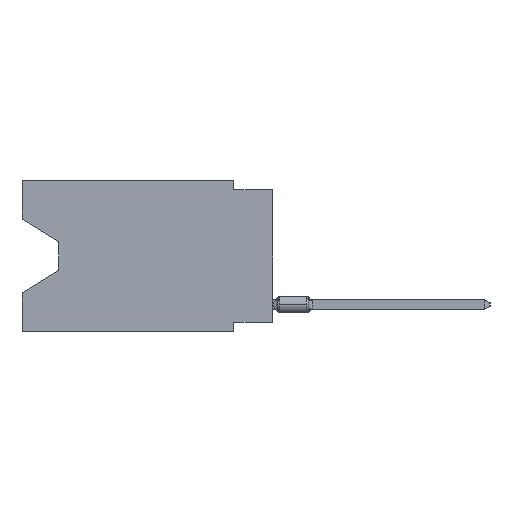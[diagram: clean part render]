
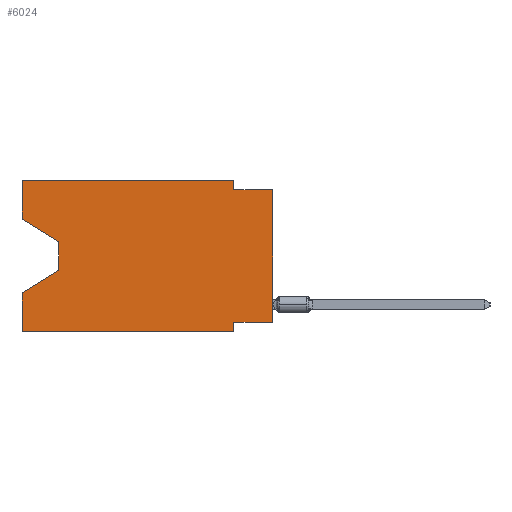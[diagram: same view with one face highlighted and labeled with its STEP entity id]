
A CAD part, left-side view. The second image highlights one B-rep face of the part: STEP entity #6024.
In plain terms, the highlighted planar face has unit normal (-1, 0, 0).
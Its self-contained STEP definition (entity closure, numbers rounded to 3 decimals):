
#334 = ORIENTED_EDGE ( 'NONE', *, *, #66144, .F. ) ;
#1323 = CARTESIAN_POINT ( 'NONE',  ( 0., 16.383, 0. ) ) ;
#2245 = VECTOR ( 'NONE', #31888, 1000. ) ;
#2262 = CARTESIAN_POINT ( 'NONE',  ( 0., 0., -9.271 ) ) ;
#2269 = CARTESIAN_POINT ( 'NONE',  ( 0., 0., -9.271 ) ) ;
#2447 = DIRECTION ( 'NONE',  ( 0., -1., 0. ) ) ;
#5478 = VECTOR ( 'NONE', #59322, 1000. ) ;
#5703 = DIRECTION ( 'NONE',  ( 0., 0.855, -0.519 ) ) ;
#5725 = EDGE_CURVE ( 'NONE', #48758, #46616, #27252, .T. ) ;
#6010 = CARTESIAN_POINT ( 'NONE',  ( 0., 2.54, 0. ) ) ;
#6024 = ADVANCED_FACE ( 'NONE', ( #52932 ), #61983, .F. ) ;
#7100 = CARTESIAN_POINT ( 'NONE',  ( 0., 16.383, -2.546 ) ) ;
#7611 = VERTEX_POINT ( 'NONE', #12089 ) ;
#8440 = CARTESIAN_POINT ( 'NONE',  ( 0., 0., 0. ) ) ;
#9444 = CARTESIAN_POINT ( 'NONE',  ( 0., 13.97, -4.013 ) ) ;
#9773 = LINE ( 'NONE', #9444, #12158 ) ;
#11030 = LINE ( 'NONE', #6010, #12050 ) ;
#11158 = CARTESIAN_POINT ( 'NONE',  ( 0., 16.383, 0. ) ) ;
#12050 = VECTOR ( 'NONE', #37472, 1000. ) ;
#12089 = CARTESIAN_POINT ( 'NONE',  ( 0., 16.383, 0. ) ) ;
#12129 = LINE ( 'NONE', #52968, #2245 ) ;
#12158 = VECTOR ( 'NONE', #35220, 1000. ) ;
#12328 = CARTESIAN_POINT ( 'NONE',  ( 0., 2.54, 0. ) ) ;
#12699 = VECTOR ( 'NONE', #32160, 1000. ) ;
#13180 = EDGE_CURVE ( 'NONE', #48758, #56253, #32831, .T. ) ;
#13791 = ORIENTED_EDGE ( 'NONE', *, *, #5725, .T. ) ;
#14421 = VERTEX_POINT ( 'NONE', #64103 ) ;
#15092 = CARTESIAN_POINT ( 'NONE',  ( 0., 13.97, -5.893 ) ) ;
#16835 = LINE ( 'NONE', #57660, #46651 ) ;
#17279 = ORIENTED_EDGE ( 'NONE', *, *, #28565, .T. ) ;
#18452 = VECTOR ( 'NONE', #57267, 1000. ) ;
#18832 = CARTESIAN_POINT ( 'NONE',  ( 0., 13.97, -5.893 ) ) ;
#19521 = VECTOR ( 'NONE', #26557, 1000. ) ;
#21091 = VERTEX_POINT ( 'NONE', #2269 ) ;
#21469 = DIRECTION ( 'NONE',  ( 0., 0., -1. ) ) ;
#21757 = DIRECTION ( 'NONE',  ( 0., 0., 1. ) ) ;
#21779 = CARTESIAN_POINT ( 'NONE',  ( 0., 2.54, -9.906 ) ) ;
#22031 = CARTESIAN_POINT ( 'NONE',  ( 0., 2.54, -9.906 ) ) ;
#22218 = VERTEX_POINT ( 'NONE', #18832 ) ;
#22545 = ORIENTED_EDGE ( 'NONE', *, *, #52375, .F. ) ;
#22743 = VECTOR ( 'NONE', #36440, 1000. ) ;
#23933 = LINE ( 'NONE', #15092, #49336 ) ;
#26557 = DIRECTION ( 'NONE',  ( 0., -1., 0. ) ) ;
#27252 = LINE ( 'NONE', #57044, #59268 ) ;
#28150 = CARTESIAN_POINT ( 'NONE',  ( 0., 16.383, 0. ) ) ;
#28548 = LINE ( 'NONE', #8440, #5478 ) ;
#28565 = EDGE_CURVE ( 'NONE', #49920, #22218, #9773, .T. ) ;
#29924 = CARTESIAN_POINT ( 'NONE',  ( 0., 2.54, -0.635 ) ) ;
#30490 = ORIENTED_EDGE ( 'NONE', *, *, #38653, .T. ) ;
#31888 = DIRECTION ( 'NONE',  ( 0., -1., 0. ) ) ;
#32160 = DIRECTION ( 'NONE',  ( 0., 0., 1. ) ) ;
#32235 = DIRECTION ( 'NONE',  ( 0., -0.855, -0.519 ) ) ;
#32514 = VERTEX_POINT ( 'NONE', #12328 ) ;
#32824 = LINE ( 'NONE', #21779, #18452 ) ;
#32831 = LINE ( 'NONE', #28150, #12699 ) ;
#32855 = CARTESIAN_POINT ( 'NONE',  ( 0., 16.383, 0. ) ) ;
#33245 = CARTESIAN_POINT ( 'NONE',  ( 0., 16.383, -9.906 ) ) ;
#35220 = DIRECTION ( 'NONE',  ( 0., 0., -1. ) ) ;
#36294 = VERTEX_POINT ( 'NONE', #7100 ) ;
#36440 = DIRECTION ( 'NONE',  ( 0., 1., 0. ) ) ;
#36730 = EDGE_CURVE ( 'NONE', #36294, #7611, #62929, .T. ) ;
#37472 = DIRECTION ( 'NONE',  ( 0., 0., -1. ) ) ;
#38653 = EDGE_CURVE ( 'NONE', #22218, #56253, #23933, .T. ) ;
#39227 = VERTEX_POINT ( 'NONE', #47815 ) ;
#40091 = ORIENTED_EDGE ( 'NONE', *, *, #44404, .F. ) ;
#42024 = ORIENTED_EDGE ( 'NONE', *, *, #59026, .T. ) ;
#42817 = EDGE_CURVE ( 'NONE', #21091, #39227, #28548, .T. ) ;
#44404 = EDGE_CURVE ( 'NONE', #14421, #46616, #32824, .T. ) ;
#44795 = EDGE_CURVE ( 'NONE', #21091, #14421, #48138, .T. ) ;
#46222 = CARTESIAN_POINT ( 'NONE',  ( 0., 13.97, -4.013 ) ) ;
#46616 = VERTEX_POINT ( 'NONE', #22031 ) ;
#46651 = VECTOR ( 'NONE', #32235, 1000. ) ;
#47815 = CARTESIAN_POINT ( 'NONE',  ( 0., 0., -0.635 ) ) ;
#48050 = ORIENTED_EDGE ( 'NONE', *, *, #36730, .F. ) ;
#48138 = LINE ( 'NONE', #2262, #22743 ) ;
#48758 = VERTEX_POINT ( 'NONE', #33245 ) ;
#49336 = VECTOR ( 'NONE', #5703, 1000. ) ;
#49920 = VERTEX_POINT ( 'NONE', #46222 ) ;
#52122 = ORIENTED_EDGE ( 'NONE', *, *, #42817, .T. ) ;
#52375 = EDGE_CURVE ( 'NONE', #7611, #32514, #57025, .T. ) ;
#52932 = FACE_OUTER_BOUND ( 'NONE', #60355, .T. ) ;
#52968 = CARTESIAN_POINT ( 'NONE',  ( 0., 0., -0.635 ) ) ;
#53418 = EDGE_CURVE ( 'NONE', #32514, #66034, #11030, .T. ) ;
#53425 = ORIENTED_EDGE ( 'NONE', *, *, #44795, .F. ) ;
#56253 = VERTEX_POINT ( 'NONE', #57818 ) ;
#57025 = LINE ( 'NONE', #11158, #19521 ) ;
#57044 = CARTESIAN_POINT ( 'NONE',  ( 0., 16.383, -9.906 ) ) ;
#57267 = DIRECTION ( 'NONE',  ( 0., 0., -1. ) ) ;
#57660 = CARTESIAN_POINT ( 'NONE',  ( 0., 16.383, -2.546 ) ) ;
#57665 = VECTOR ( 'NONE', #21757, 1000. ) ;
#57818 = CARTESIAN_POINT ( 'NONE',  ( 0., 16.383, -7.36 ) ) ;
#59026 = EDGE_CURVE ( 'NONE', #36294, #49920, #16835, .T. ) ;
#59268 = VECTOR ( 'NONE', #2447, 1000. ) ;
#59322 = DIRECTION ( 'NONE',  ( 0., 0., 1. ) ) ;
#60355 = EDGE_LOOP ( 'NONE', ( #42024, #17279, #30490, #64812, #13791, #40091, #53425, #52122, #334, #62747, #22545, #48050 ) ) ;
#61983 = PLANE ( 'NONE',  #64672 ) ;
#62747 = ORIENTED_EDGE ( 'NONE', *, *, #53418, .F. ) ;
#62929 = LINE ( 'NONE', #1323, #57665 ) ;
#62977 = DIRECTION ( 'NONE',  ( 1., 0., 0. ) ) ;
#64103 = CARTESIAN_POINT ( 'NONE',  ( 0., 2.54, -9.271 ) ) ;
#64672 = AXIS2_PLACEMENT_3D ( 'NONE', #32855, #62977, #21469 ) ;
#64812 = ORIENTED_EDGE ( 'NONE', *, *, #13180, .F. ) ;
#66034 = VERTEX_POINT ( 'NONE', #29924 ) ;
#66144 = EDGE_CURVE ( 'NONE', #66034, #39227, #12129, .T. ) ;
